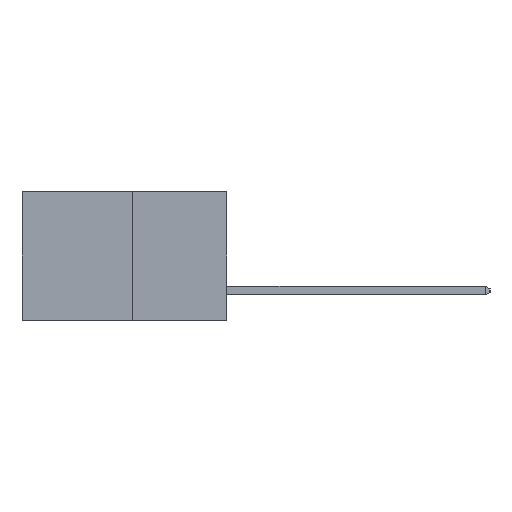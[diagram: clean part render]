
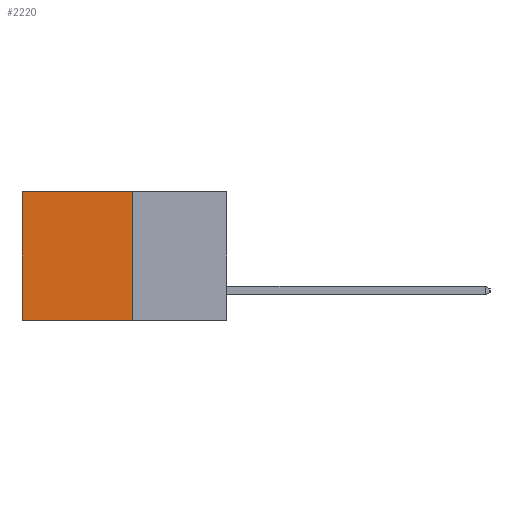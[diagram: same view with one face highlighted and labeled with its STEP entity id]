
A CAD part, left-side view. The second image highlights one B-rep face of the part: STEP entity #2220.
In plain terms, the highlighted planar face has unit normal (-1, 0, 0).
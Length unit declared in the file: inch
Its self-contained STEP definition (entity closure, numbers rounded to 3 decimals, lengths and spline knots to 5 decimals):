
#24 = LINE ( 'NONE', #6650, #5902 ) ;
#267 = VERTEX_POINT ( 'NONE', #3874 ) ;
#300 = PLANE ( 'NONE',  #8768 ) ;
#967 = EDGE_CURVE ( 'NONE', #6067, #8081, #3397, .T. ) ;
#1109 = DIRECTION ( 'NONE',  ( 0., 0., -1. ) ) ;
#2220 = ADVANCED_FACE ( 'NONE', ( #3193 ), #300, .F. ) ;
#2256 = DIRECTION ( 'NONE',  ( 1., 0., 0. ) ) ;
#2742 = EDGE_LOOP ( 'NONE', ( #3623, #3754, #3824, #3966 ) ) ;
#2919 = CARTESIAN_POINT ( 'NONE',  ( 0.277, 0.27, -0.37 ) ) ;
#3052 = CARTESIAN_POINT ( 'NONE',  ( 0.277, 0.27, -0.37 ) ) ;
#3193 = FACE_OUTER_BOUND ( 'NONE', #2742, .T. ) ;
#3397 = LINE ( 'NONE', #3052, #7258 ) ;
#3623 = ORIENTED_EDGE ( 'NONE', *, *, #8209, .T. ) ;
#3754 = ORIENTED_EDGE ( 'NONE', *, *, #5784, .F. ) ;
#3824 = ORIENTED_EDGE ( 'NONE', *, *, #967, .F. ) ;
#3874 = CARTESIAN_POINT ( 'NONE',  ( 0.277, 0.59, 0. ) ) ;
#3894 = CARTESIAN_POINT ( 'NONE',  ( 0.277, 0.59, -0.37 ) ) ;
#3966 = ORIENTED_EDGE ( 'NONE', *, *, #5111, .T. ) ;
#4024 = DIRECTION ( 'NONE',  ( 0., 0., -1. ) ) ;
#4474 = VECTOR ( 'NONE', #4024, 39.37008 ) ;
#4740 = CARTESIAN_POINT ( 'NONE',  ( 0.277, 0.27, -0.37 ) ) ;
#5111 = EDGE_CURVE ( 'NONE', #6067, #267, #24, .T. ) ;
#5133 = VECTOR ( 'NONE', #9513, 39.37008 ) ;
#5501 = DIRECTION ( 'NONE',  ( 0., 0., -1. ) ) ;
#5784 = EDGE_CURVE ( 'NONE', #8081, #5886, #7216, .T. ) ;
#5886 = VERTEX_POINT ( 'NONE', #8751 ) ;
#5902 = VECTOR ( 'NONE', #6097, 39.37008 ) ;
#6067 = VERTEX_POINT ( 'NONE', #7534 ) ;
#6097 = DIRECTION ( 'NONE',  ( 0., 1., 0. ) ) ;
#6650 = CARTESIAN_POINT ( 'NONE',  ( 0.277, 0.27, 0. ) ) ;
#7216 = LINE ( 'NONE', #9422, #5133 ) ;
#7258 = VECTOR ( 'NONE', #1109, 39.37008 ) ;
#7534 = CARTESIAN_POINT ( 'NONE',  ( 0.277, 0.27, 0. ) ) ;
#8081 = VERTEX_POINT ( 'NONE', #4740 ) ;
#8209 = EDGE_CURVE ( 'NONE', #267, #5886, #8478, .T. ) ;
#8478 = LINE ( 'NONE', #3894, #4474 ) ;
#8751 = CARTESIAN_POINT ( 'NONE',  ( 0.277, 0.59, -0.37 ) ) ;
#8768 = AXIS2_PLACEMENT_3D ( 'NONE', #2919, #2256, #5501 ) ;
#9422 = CARTESIAN_POINT ( 'NONE',  ( 0.277, 0.27, -0.37 ) ) ;
#9513 = DIRECTION ( 'NONE',  ( 0., 1., 0. ) ) ;
